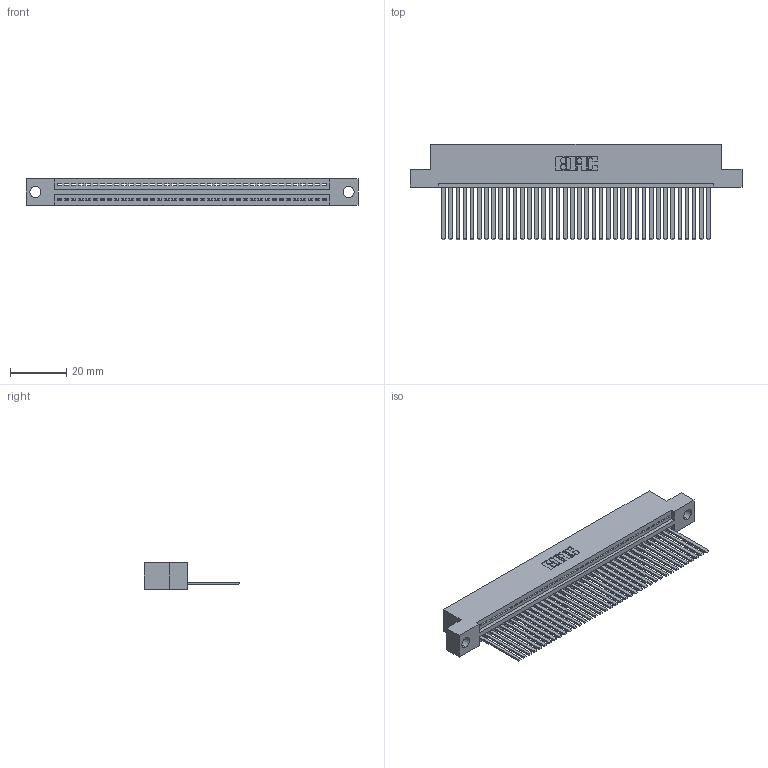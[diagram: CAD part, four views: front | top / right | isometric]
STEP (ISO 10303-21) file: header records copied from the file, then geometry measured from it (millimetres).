
FILE_DESCRIPTION (( 'STEP AP203' ), '1' );
FILE_NAME ('395-038-544-104.STEP', '2018-11-14T05:09:23', ( '' ), ( '' ), 'SwSTEP 2.0', 'SolidWorks 2016', '' );
FILE_SCHEMA (( 'CONFIG_CONTROL_DESIGN' ));
Length unit declared in the file: inch
Products named in the file (3): 345 Part_Flush Mounting Lugs - 0.156 Dia-TH; 395-038-544-104; 345-292-001_345-293-144
Assembly tree (39 placements, depth 2):
  395-038-544-104
    345 Part_Flush Mounting Lugs - 0.156 Dia-TH
    345-292-001_345-293-144  x38
Bounding box: 117.73 x 33.96 x 9.4 mm (x, y, z)
Volume: 11501.5 mm3; surface area: 16360 mm2
Topology: 39 solids, 39 shells, 2102 faces, 6345 edges, 4178 vertices
Faces by surface type: plane 1448, cylinder 654
Entity records: 28957 total; most frequent: CARTESIAN_POINT 5022, ORIENTED_EDGE 4994, DIRECTION 4389, EDGE_CURVE 2497, VECTOR 2217, LINE 2217, VERTEX_POINT 1662, AXIS2_PLACEMENT_3D 1086
